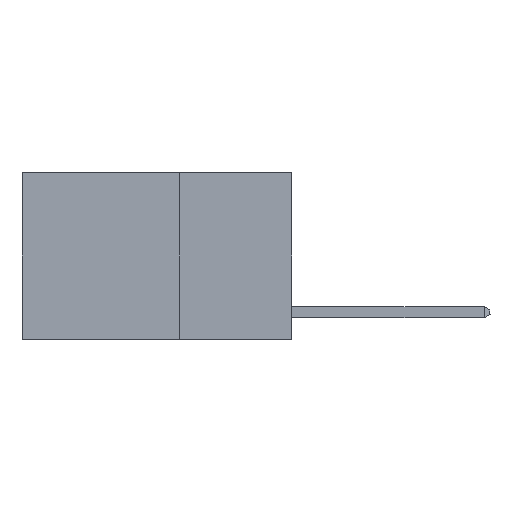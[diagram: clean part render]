
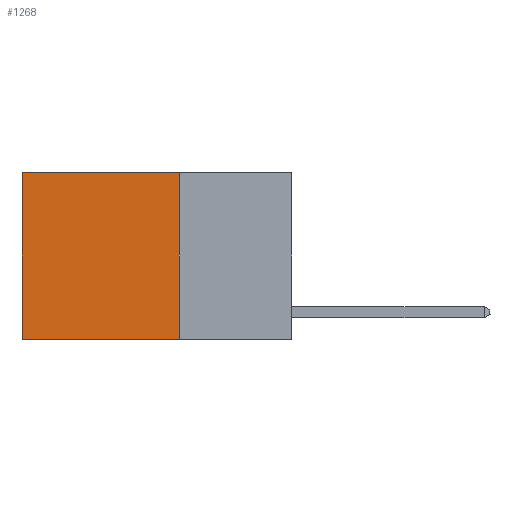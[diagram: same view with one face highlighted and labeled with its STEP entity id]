
A CAD part, left-side view. The second image highlights one B-rep face of the part: STEP entity #1268.
In plain terms, the highlighted planar face has unit normal (-1, 0, 0).
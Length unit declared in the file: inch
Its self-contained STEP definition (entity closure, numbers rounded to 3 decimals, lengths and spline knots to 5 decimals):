
#1116 = LINE ( 'NONE', #3367, #5083 ) ;
#1268 = ADVANCED_FACE ( 'NONE', ( #1972 ), #3516, .F. ) ;
#1599 = VECTOR ( 'NONE', #7304, 39.37008 ) ;
#1610 = LINE ( 'NONE', #9027, #6443 ) ;
#1879 = DIRECTION ( 'NONE',  ( 0., 0., -1. ) ) ;
#1928 = CARTESIAN_POINT ( 'NONE',  ( 0.2625, 0.25, 0. ) ) ;
#1972 = FACE_OUTER_BOUND ( 'NONE', #9212, .T. ) ;
#2375 = EDGE_CURVE ( 'NONE', #6801, #3997, #1116, .T. ) ;
#2457 = VECTOR ( 'NONE', #7576, 39.37008 ) ;
#2645 = CARTESIAN_POINT ( 'NONE',  ( 0.2625, 0.6, -0.37 ) ) ;
#2671 = CARTESIAN_POINT ( 'NONE',  ( 0.2625, 0.25, 0. ) ) ;
#2886 = CARTESIAN_POINT ( 'NONE',  ( 0.2625, 0.25, -0.37 ) ) ;
#3239 = EDGE_CURVE ( 'NONE', #5186, #7021, #4512, .T. ) ;
#3367 = CARTESIAN_POINT ( 'NONE',  ( 0.2625, 0.25, 0. ) ) ;
#3516 = PLANE ( 'NONE',  #5227 ) ;
#3997 = VERTEX_POINT ( 'NONE', #5502 ) ;
#4307 = ORIENTED_EDGE ( 'NONE', *, *, #2375, .T. ) ;
#4512 = LINE ( 'NONE', #2886, #1599 ) ;
#4542 = DIRECTION ( 'NONE',  ( 0., 0., -1. ) ) ;
#5083 = VECTOR ( 'NONE', #9217, 39.37008 ) ;
#5186 = VERTEX_POINT ( 'NONE', #7869 ) ;
#5227 = AXIS2_PLACEMENT_3D ( 'NONE', #1928, #7110, #1879 ) ;
#5494 = LINE ( 'NONE', #6836, #2457 ) ;
#5502 = CARTESIAN_POINT ( 'NONE',  ( 0.2625, 0.6, 0. ) ) ;
#5533 = EDGE_CURVE ( 'NONE', #6801, #5186, #1610, .T. ) ;
#6443 = VECTOR ( 'NONE', #4542, 39.37008 ) ;
#6518 = ORIENTED_EDGE ( 'NONE', *, *, #5533, .F. ) ;
#6744 = EDGE_CURVE ( 'NONE', #3997, #7021, #5494, .T. ) ;
#6801 = VERTEX_POINT ( 'NONE', #2671 ) ;
#6836 = CARTESIAN_POINT ( 'NONE',  ( 0.2625, 0.6, 0. ) ) ;
#7021 = VERTEX_POINT ( 'NONE', #2645 ) ;
#7110 = DIRECTION ( 'NONE',  ( 1., 0., 0. ) ) ;
#7304 = DIRECTION ( 'NONE',  ( 0., 1., 0. ) ) ;
#7518 = ORIENTED_EDGE ( 'NONE', *, *, #6744, .T. ) ;
#7576 = DIRECTION ( 'NONE',  ( 0., 0., -1. ) ) ;
#7869 = CARTESIAN_POINT ( 'NONE',  ( 0.2625, 0.25, -0.37 ) ) ;
#8762 = ORIENTED_EDGE ( 'NONE', *, *, #3239, .F. ) ;
#9027 = CARTESIAN_POINT ( 'NONE',  ( 0.2625, 0.25, 0. ) ) ;
#9212 = EDGE_LOOP ( 'NONE', ( #7518, #8762, #6518, #4307 ) ) ;
#9217 = DIRECTION ( 'NONE',  ( 0., 1., 0. ) ) ;
